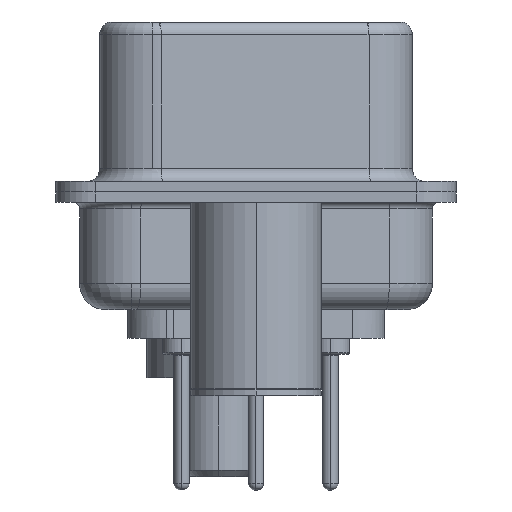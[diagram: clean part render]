
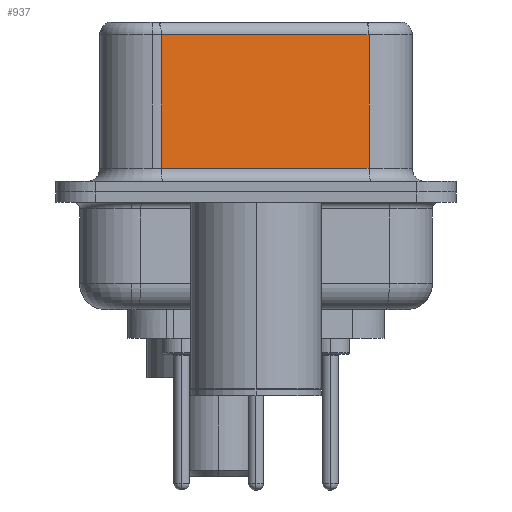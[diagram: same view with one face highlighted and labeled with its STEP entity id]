
A CAD part, left-side view. The second image highlights one B-rep face of the part: STEP entity #937.
In plain terms, the highlighted planar face has unit normal (-0.985, -0.174, 0).
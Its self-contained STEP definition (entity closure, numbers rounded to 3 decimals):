
#771 = CARTESIAN_POINT ( 'NONE',  ( 3.73, 3.628, 6.52 ) ) ;
#937 = ADVANCED_FACE ( 'NONE', ( #15622 ), #13047, .F. ) ;
#1019 = EDGE_CURVE ( 'NONE', #19440, #19059, #25390, .T. ) ;
#4400 = ORIENTED_EDGE ( 'NONE', *, *, #4719, .T. ) ;
#4457 = DIRECTION ( 'NONE',  ( -0.174, 0.985, 0. ) ) ;
#4719 = EDGE_CURVE ( 'NONE', #6792, #6043, #22117, .T. ) ;
#6043 = VERTEX_POINT ( 'NONE', #22471 ) ;
#6355 = DIRECTION ( 'NONE',  ( -0.174, 0.985, 0. ) ) ;
#6792 = VERTEX_POINT ( 'NONE', #14906 ) ;
#7210 = CARTESIAN_POINT ( 'NONE',  ( 5.132, -4.322, 6.02 ) ) ;
#7364 = VECTOR ( 'NONE', #15342, 1000. ) ;
#11766 = CARTESIAN_POINT ( 'NONE',  ( 5.132, -4.322, 6.52 ) ) ;
#12932 = DIRECTION ( 'NONE',  ( 0.985, 0.174, 0. ) ) ;
#13043 = LINE ( 'NONE', #771, #24266 ) ;
#13047 = PLANE ( 'NONE',  #27246 ) ;
#14906 = CARTESIAN_POINT ( 'NONE',  ( 3.73, 3.628, 0.9 ) ) ;
#15037 = CARTESIAN_POINT ( 'NONE',  ( 5.132, -4.322, 0.9 ) ) ;
#15154 = ORIENTED_EDGE ( 'NONE', *, *, #20342, .F. ) ;
#15342 = DIRECTION ( 'NONE',  ( 0.174, -0.985, 0. ) ) ;
#15622 = FACE_OUTER_BOUND ( 'NONE', #28878, .T. ) ;
#18631 = EDGE_CURVE ( 'NONE', #19059, #6792, #13043, .T. ) ;
#19059 = VERTEX_POINT ( 'NONE', #22542 ) ;
#19440 = VERTEX_POINT ( 'NONE', #7210 ) ;
#19528 = ORIENTED_EDGE ( 'NONE', *, *, #1019, .T. ) ;
#20342 = EDGE_CURVE ( 'NONE', #19440, #6043, #24215, .T. ) ;
#21101 = DIRECTION ( 'NONE',  ( 0., 0., -1. ) ) ;
#21401 = DIRECTION ( 'NONE',  ( 0., 0., -1. ) ) ;
#22117 = LINE ( 'NONE', #15037, #7364 ) ;
#22471 = CARTESIAN_POINT ( 'NONE',  ( 5.132, -4.322, 0.9 ) ) ;
#22542 = CARTESIAN_POINT ( 'NONE',  ( 3.73, 3.628, 6.02 ) ) ;
#22831 = ORIENTED_EDGE ( 'NONE', *, *, #18631, .T. ) ;
#23514 = VECTOR ( 'NONE', #21401, 1000. ) ;
#24215 = LINE ( 'NONE', #25860, #23514 ) ;
#24266 = VECTOR ( 'NONE', #21101, 1000. ) ;
#25390 = LINE ( 'NONE', #28169, #26079 ) ;
#25860 = CARTESIAN_POINT ( 'NONE',  ( 5.132, -4.322, 6.52 ) ) ;
#26079 = VECTOR ( 'NONE', #4457, 1000. ) ;
#27246 = AXIS2_PLACEMENT_3D ( 'NONE', #11766, #12932, #6355 ) ;
#28169 = CARTESIAN_POINT ( 'NONE',  ( 5.132, -4.322, 6.02 ) ) ;
#28878 = EDGE_LOOP ( 'NONE', ( #15154, #19528, #22831, #4400 ) ) ;
